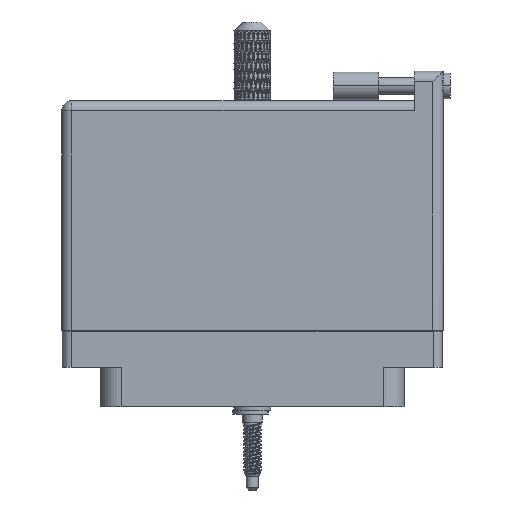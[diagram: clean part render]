
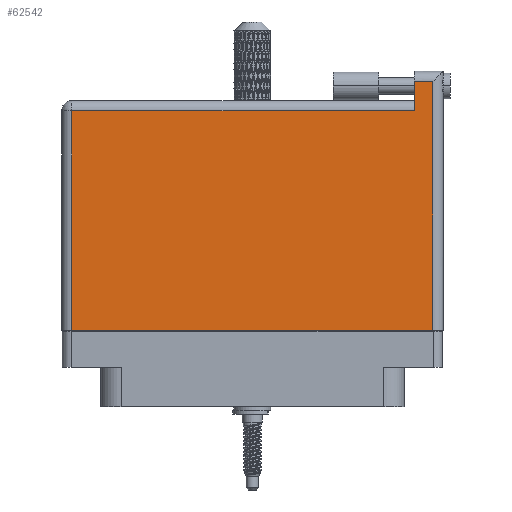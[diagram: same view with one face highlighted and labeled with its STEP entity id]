
A CAD part, front view. The second image highlights one B-rep face of the part: STEP entity #62542.
In plain terms, the highlighted face is planar.
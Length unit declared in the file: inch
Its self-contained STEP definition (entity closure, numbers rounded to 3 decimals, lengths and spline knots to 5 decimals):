
#3492 = DIRECTION ( 'NONE',  ( 0., 1., 0. ) ) ;
#5999 = VERTEX_POINT ( 'NONE', #49325 ) ;
#12745 = CARTESIAN_POINT ( 'NONE',  ( 1.103, 1.666, 0.4495 ) ) ;
#18757 = DIRECTION ( 'NONE',  ( -1., 0., 0. ) ) ;
#20598 = CARTESIAN_POINT ( 'NONE',  ( 1.23, 1.666, 0.4495 ) ) ;
#20658 = CARTESIAN_POINT ( 'NONE',  ( -1.3, -0.1, 0.4495 ) ) ;
#22261 = CARTESIAN_POINT ( 'NONE',  ( -1.3, 1.466, 0.4495 ) ) ;
#24539 = VERTEX_POINT ( 'NONE', #89115 ) ;
#24649 = EDGE_CURVE ( 'NONE', #24539, #66206, #73499, .T. ) ;
#24937 = CARTESIAN_POINT ( 'NONE',  ( 1.23, 1.596, 0.4495 ) ) ;
#32007 = EDGE_CURVE ( 'NONE', #107780, #51691, #71916, .T. ) ;
#32189 = EDGE_CURVE ( 'NONE', #5999, #107780, #104317, .T. ) ;
#41087 = LINE ( 'NONE', #81346, #48105 ) ;
#41362 = VECTOR ( 'NONE', #48395, 39.37008 ) ;
#41792 = ORIENTED_EDGE ( 'NONE', *, *, #24649, .T. ) ;
#42658 = LINE ( 'NONE', #20658, #41362 ) ;
#47688 = DIRECTION ( 'NONE',  ( 0., -1., 0. ) ) ;
#48105 = VECTOR ( 'NONE', #18757, 39.37008 ) ;
#48395 = DIRECTION ( 'NONE',  ( 1., 0., 0. ) ) ;
#49325 = CARTESIAN_POINT ( 'NONE',  ( 1.103, 1.596, 0.4495 ) ) ;
#51691 = VERTEX_POINT ( 'NONE', #63879 ) ;
#51748 = CARTESIAN_POINT ( 'NONE',  ( -1.23, -0.1, 0.4495 ) ) ;
#62500 = VERTEX_POINT ( 'NONE', #66300 ) ;
#62542 = ADVANCED_FACE ( 'NONE', ( #72566 ), #84074, .F. ) ;
#63879 = CARTESIAN_POINT ( 'NONE',  ( -1.23, 1.396, 0.4495 ) ) ;
#64345 = EDGE_CURVE ( 'NONE', #51691, #62500, #111941, .T. ) ;
#65629 = CARTESIAN_POINT ( 'NONE',  ( 1.103, 1.396, 0.4495 ) ) ;
#66206 = VERTEX_POINT ( 'NONE', #24937 ) ;
#66300 = CARTESIAN_POINT ( 'NONE',  ( -1.23, -0.1, 0.4495 ) ) ;
#66669 = VECTOR ( 'NONE', #88150, 39.37008 ) ;
#67851 = DIRECTION ( 'NONE',  ( -1., 0., 0. ) ) ;
#71916 = LINE ( 'NONE', #97953, #110150 ) ;
#72566 = FACE_OUTER_BOUND ( 'NONE', #95624, .T. ) ;
#73499 = LINE ( 'NONE', #20598, #100371 ) ;
#77983 = ORIENTED_EDGE ( 'NONE', *, *, #88882, .T. ) ;
#78886 = VECTOR ( 'NONE', #47688, 39.37008 ) ;
#81346 = CARTESIAN_POINT ( 'NONE',  ( -1.3, 1.596, 0.4495 ) ) ;
#82338 = ORIENTED_EDGE ( 'NONE', *, *, #32189, .T. ) ;
#84074 = PLANE ( 'NONE',  #97999 ) ;
#88150 = DIRECTION ( 'NONE',  ( 0., -1., 0. ) ) ;
#88882 = EDGE_CURVE ( 'NONE', #66206, #5999, #41087, .T. ) ;
#89115 = CARTESIAN_POINT ( 'NONE',  ( 1.23, -0.1, 0.4495 ) ) ;
#92556 = EDGE_CURVE ( 'NONE', #62500, #24539, #42658, .T. ) ;
#93976 = DIRECTION ( 'NONE',  ( 0., 0., -1. ) ) ;
#94007 = ORIENTED_EDGE ( 'NONE', *, *, #64345, .T. ) ;
#95624 = EDGE_LOOP ( 'NONE', ( #102337, #41792, #77983, #82338, #116380, #94007 ) ) ;
#97953 = CARTESIAN_POINT ( 'NONE',  ( -1.3, 1.396, 0.4495 ) ) ;
#97999 = AXIS2_PLACEMENT_3D ( 'NONE', #22261, #93976, #67851 ) ;
#100371 = VECTOR ( 'NONE', #3492, 39.37008 ) ;
#102337 = ORIENTED_EDGE ( 'NONE', *, *, #92556, .T. ) ;
#104317 = LINE ( 'NONE', #12745, #78886 ) ;
#107780 = VERTEX_POINT ( 'NONE', #65629 ) ;
#108216 = DIRECTION ( 'NONE',  ( -1., 0., 0. ) ) ;
#110150 = VECTOR ( 'NONE', #108216, 39.37008 ) ;
#111941 = LINE ( 'NONE', #51748, #66669 ) ;
#116380 = ORIENTED_EDGE ( 'NONE', *, *, #32007, .T. ) ;
